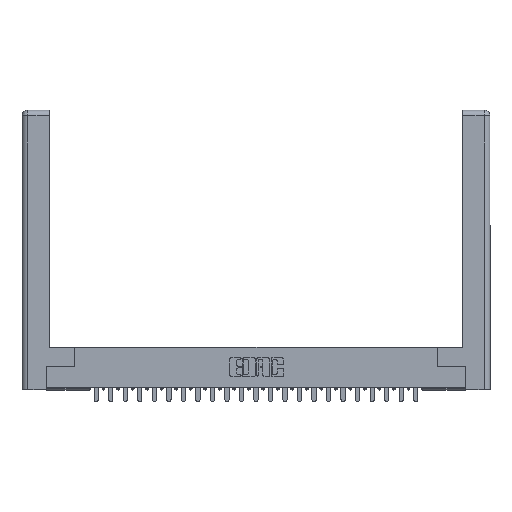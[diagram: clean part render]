
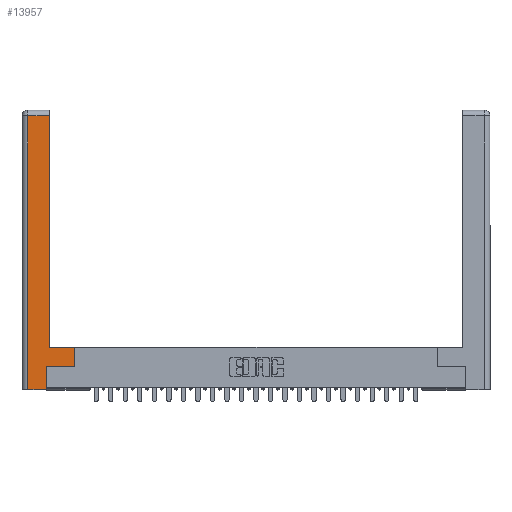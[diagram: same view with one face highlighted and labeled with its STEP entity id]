
A CAD part, top view. The second image highlights one B-rep face of the part: STEP entity #13957.
In plain terms, the highlighted planar face has unit normal (0, 0, 1).
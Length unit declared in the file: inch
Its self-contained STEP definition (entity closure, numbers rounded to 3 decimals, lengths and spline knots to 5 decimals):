
#30 = VERTEX_POINT ( 'NONE', #2775 ) ;
#406 = VECTOR ( 'NONE', #6108, 39.37008 ) ;
#443 = LINE ( 'NONE', #19359, #4110 ) ;
#553 = DIRECTION ( 'NONE',  ( 1., 0., 0. ) ) ;
#1512 = CARTESIAN_POINT ( 'NONE',  ( 0.565, 0.245, 0. ) ) ;
#1940 = ORIENTED_EDGE ( 'NONE', *, *, #27122, .T. ) ;
#1942 = DIRECTION ( 'NONE',  ( -1., 0., 0. ) ) ;
#1998 = AXIS2_PLACEMENT_3D ( 'NONE', #20059, #15539, #1942 ) ;
#2126 = EDGE_CURVE ( 'NONE', #21407, #17033, #443, .T. ) ;
#2448 = EDGE_CURVE ( 'NONE', #8380, #27643, #18431, .T. ) ;
#2501 = CARTESIAN_POINT ( 'NONE',  ( 0.565, 0.45, 0. ) ) ;
#2775 = CARTESIAN_POINT ( 'NONE',  ( 0.0615, 2.94, 0. ) ) ;
#2925 = ORIENTED_EDGE ( 'NONE', *, *, #2126, .T. ) ;
#4110 = VECTOR ( 'NONE', #21980, 39.37008 ) ;
#4362 = EDGE_CURVE ( 'NONE', #17033, #12304, #28724, .T. ) ;
#6108 = DIRECTION ( 'NONE',  ( -1., 0., 0. ) ) ;
#6164 = DIRECTION ( 'NONE',  ( 0., 1., 0. ) ) ;
#6499 = CARTESIAN_POINT ( 'NONE',  ( 0.265, 0.245, 0. ) ) ;
#6540 = DIRECTION ( 'NONE',  ( 0., -1., 0. ) ) ;
#7232 = VECTOR ( 'NONE', #6540, 39.37008 ) ;
#7328 = LINE ( 'NONE', #28312, #10553 ) ;
#7419 = VERTEX_POINT ( 'NONE', #24170 ) ;
#8029 = VECTOR ( 'NONE', #6164, 39.37008 ) ;
#8175 = CARTESIAN_POINT ( 'NONE',  ( 0.295, 0.45, 0. ) ) ;
#8380 = VERTEX_POINT ( 'NONE', #18765 ) ;
#9870 = CARTESIAN_POINT ( 'NONE',  ( 0.265, 0., 0. ) ) ;
#10213 = DIRECTION ( 'NONE',  ( -1., 0., 0. ) ) ;
#10538 = LINE ( 'NONE', #8175, #406 ) ;
#10553 = VECTOR ( 'NONE', #10213, 39.37008 ) ;
#10723 = VECTOR ( 'NONE', #553, 39.37008 ) ;
#10727 = ORIENTED_EDGE ( 'NONE', *, *, #24976, .T. ) ;
#11113 = EDGE_CURVE ( 'NONE', #27643, #30, #7328, .T. ) ;
#11413 = ORIENTED_EDGE ( 'NONE', *, *, #4362, .T. ) ;
#12304 = VERTEX_POINT ( 'NONE', #2501 ) ;
#12543 = LINE ( 'NONE', #23581, #16825 ) ;
#12800 = ORIENTED_EDGE ( 'NONE', *, *, #11113, .T. ) ;
#13762 = CARTESIAN_POINT ( 'NONE',  ( 0.0615, 0., 0. ) ) ;
#13957 = ADVANCED_FACE ( 'NONE', ( #26286 ), #29440, .F. ) ;
#14185 = DIRECTION ( 'NONE',  ( 0., 1., 0. ) ) ;
#14250 = EDGE_CURVE ( 'NONE', #12304, #8380, #10538, .T. ) ;
#14281 = ORIENTED_EDGE ( 'NONE', *, *, #2448, .T. ) ;
#15129 = VECTOR ( 'NONE', #21289, 39.37008 ) ;
#15492 = VERTEX_POINT ( 'NONE', #13762 ) ;
#15539 = DIRECTION ( 'NONE',  ( 0., 0., -1. ) ) ;
#16825 = VECTOR ( 'NONE', #14185, 39.37008 ) ;
#16917 = CARTESIAN_POINT ( 'NONE',  ( 0.295, 3., 0. ) ) ;
#17033 = VERTEX_POINT ( 'NONE', #1512 ) ;
#18340 = LINE ( 'NONE', #29371, #7232 ) ;
#18431 = LINE ( 'NONE', #16917, #8029 ) ;
#18765 = CARTESIAN_POINT ( 'NONE',  ( 0.295, 0.45, 0. ) ) ;
#19359 = CARTESIAN_POINT ( 'NONE',  ( 0.565, 0.245, 0. ) ) ;
#20059 = CARTESIAN_POINT ( 'NONE',  ( 0., 0., 0. ) ) ;
#20316 = EDGE_LOOP ( 'NONE', ( #14281, #12800, #10727, #1940, #21722, #2925, #11413, #25544 ) ) ;
#21289 = DIRECTION ( 'NONE',  ( 0., 1., 0. ) ) ;
#21407 = VERTEX_POINT ( 'NONE', #6499 ) ;
#21672 = CARTESIAN_POINT ( 'NONE',  ( 0.565, 0.45, 0. ) ) ;
#21722 = ORIENTED_EDGE ( 'NONE', *, *, #25547, .T. ) ;
#21980 = DIRECTION ( 'NONE',  ( 1., 0., 0. ) ) ;
#23581 = CARTESIAN_POINT ( 'NONE',  ( 0.265, 0.245, 0. ) ) ;
#24170 = CARTESIAN_POINT ( 'NONE',  ( 0.265, 0., 0. ) ) ;
#24976 = EDGE_CURVE ( 'NONE', #30, #15492, #18340, .T. ) ;
#25544 = ORIENTED_EDGE ( 'NONE', *, *, #14250, .T. ) ;
#25547 = EDGE_CURVE ( 'NONE', #7419, #21407, #12543, .T. ) ;
#26286 = FACE_OUTER_BOUND ( 'NONE', #20316, .T. ) ;
#27122 = EDGE_CURVE ( 'NONE', #15492, #7419, #27882, .T. ) ;
#27643 = VERTEX_POINT ( 'NONE', #28799 ) ;
#27882 = LINE ( 'NONE', #9870, #10723 ) ;
#28312 = CARTESIAN_POINT ( 'NONE',  ( 0.0615, 2.94, 0. ) ) ;
#28724 = LINE ( 'NONE', #21672, #15129 ) ;
#28799 = CARTESIAN_POINT ( 'NONE',  ( 0.295, 2.94, 0. ) ) ;
#29371 = CARTESIAN_POINT ( 'NONE',  ( 0.0615, 0., 0. ) ) ;
#29440 = PLANE ( 'NONE',  #1998 ) ;
